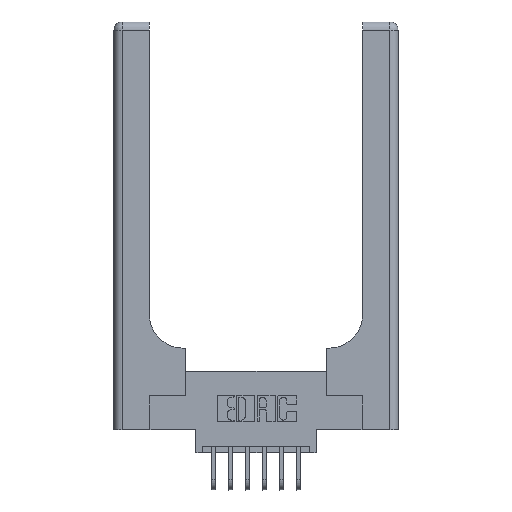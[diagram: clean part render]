
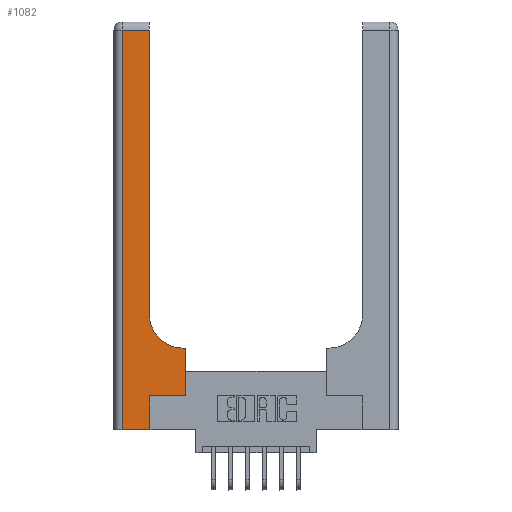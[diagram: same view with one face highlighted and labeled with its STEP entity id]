
A CAD part, top view. The second image highlights one B-rep face of the part: STEP entity #1082.
In plain terms, the highlighted planar face has unit normal (0, 0, 1).
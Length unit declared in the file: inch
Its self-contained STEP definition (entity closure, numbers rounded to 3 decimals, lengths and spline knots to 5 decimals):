
#309 = DIRECTION ( 'NONE',  ( 0., 1., 0. ) ) ;
#491 = VERTEX_POINT ( 'NONE', #1071 ) ;
#623 = CARTESIAN_POINT ( 'NONE',  ( 0.26, 0.6, 0.37 ) ) ;
#721 = VERTEX_POINT ( 'NONE', #13279 ) ;
#834 = VERTEX_POINT ( 'NONE', #8937 ) ;
#1071 = CARTESIAN_POINT ( 'NONE',  ( 0.265, 0., 0.37 ) ) ;
#1082 = ADVANCED_FACE ( 'NONE', ( #6089 ), #9531, .F. ) ;
#1418 = EDGE_CURVE ( 'NONE', #7319, #491, #8846, .T. ) ;
#1463 = CARTESIAN_POINT ( 'NONE',  ( 0.06, 0., 0.37 ) ) ;
#1487 = VERTEX_POINT ( 'NONE', #11253 ) ;
#1862 = LINE ( 'NONE', #623, #5263 ) ;
#1983 = DIRECTION ( 'NONE',  ( 0., 1., 0. ) ) ;
#2065 = ORIENTED_EDGE ( 'NONE', *, *, #6370, .T. ) ;
#2324 = CARTESIAN_POINT ( 'NONE',  ( 0., 0., 0.37 ) ) ;
#2545 = LINE ( 'NONE', #10691, #12648 ) ;
#2565 = CARTESIAN_POINT ( 'NONE',  ( 0.26, 2.94, 0.37 ) ) ;
#2700 = CARTESIAN_POINT ( 'NONE',  ( 0.51, 0.85, 0.37 ) ) ;
#2993 = VECTOR ( 'NONE', #1983, 39.37008 ) ;
#3529 = EDGE_LOOP ( 'NONE', ( #7942, #12795, #2065, #12163, #14147, #13227, #5135, #6977, #7064 ) ) ;
#3556 = EDGE_CURVE ( 'NONE', #11190, #4282, #9987, .T. ) ;
#3910 = CARTESIAN_POINT ( 'NONE',  ( 0., 2.94, 0.37 ) ) ;
#4066 = AXIS2_PLACEMENT_3D ( 'NONE', #2700, #4869, #8284 ) ;
#4282 = VERTEX_POINT ( 'NONE', #2565 ) ;
#4548 = CARTESIAN_POINT ( 'NONE',  ( 0.265, 0.25, 0.37 ) ) ;
#4570 = CARTESIAN_POINT ( 'NONE',  ( 0.26, 0.85, 0.37 ) ) ;
#4713 = EDGE_CURVE ( 'NONE', #12935, #13186, #2545, .T. ) ;
#4869 = DIRECTION ( 'NONE',  ( 0., 0., -1. ) ) ;
#5038 = DIRECTION ( 'NONE',  ( -1., 0., 0. ) ) ;
#5135 = ORIENTED_EDGE ( 'NONE', *, *, #11935, .T. ) ;
#5233 = LINE ( 'NONE', #7422, #2993 ) ;
#5263 = VECTOR ( 'NONE', #5038, 39.37008 ) ;
#5474 = DIRECTION ( 'NONE',  ( 0., 1., 0. ) ) ;
#5611 = VECTOR ( 'NONE', #14359, 39.37008 ) ;
#5801 = LINE ( 'NONE', #12477, #6898 ) ;
#5867 = CARTESIAN_POINT ( 'NONE',  ( 0., 3., 0.37 ) ) ;
#6089 = FACE_OUTER_BOUND ( 'NONE', #3529, .T. ) ;
#6301 = VECTOR ( 'NONE', #5474, 39.37008 ) ;
#6370 = EDGE_CURVE ( 'NONE', #1487, #7319, #9375, .T. ) ;
#6407 = EDGE_CURVE ( 'NONE', #721, #11190, #8878, .T. ) ;
#6898 = VECTOR ( 'NONE', #309, 39.37008 ) ;
#6977 = ORIENTED_EDGE ( 'NONE', *, *, #10795, .T. ) ;
#7064 = ORIENTED_EDGE ( 'NONE', *, *, #6407, .T. ) ;
#7268 = CARTESIAN_POINT ( 'NONE',  ( 0.06, 3., 0.37 ) ) ;
#7319 = VERTEX_POINT ( 'NONE', #1463 ) ;
#7422 = CARTESIAN_POINT ( 'NONE',  ( 0.265, 0., 0.37 ) ) ;
#7942 = ORIENTED_EDGE ( 'NONE', *, *, #3556, .T. ) ;
#8284 = DIRECTION ( 'NONE',  ( 1., 0., 0. ) ) ;
#8568 = AXIS2_PLACEMENT_3D ( 'NONE', #5867, #14009, #10554 ) ;
#8846 = LINE ( 'NONE', #2324, #5611 ) ;
#8878 = CIRCLE ( 'NONE', #4066, 0.25 ) ;
#8937 = CARTESIAN_POINT ( 'NONE',  ( 0.528, 0.6, 0.37 ) ) ;
#9375 = LINE ( 'NONE', #7268, #10310 ) ;
#9495 = DIRECTION ( 'NONE',  ( -1., 0., 0. ) ) ;
#9531 = PLANE ( 'NONE',  #8568 ) ;
#9631 = LINE ( 'NONE', #3910, #12496 ) ;
#9987 = LINE ( 'NONE', #12064, #6301 ) ;
#10310 = VECTOR ( 'NONE', #13935, 39.37008 ) ;
#10384 = EDGE_CURVE ( 'NONE', #4282, #1487, #9631, .T. ) ;
#10554 = DIRECTION ( 'NONE',  ( -1., 0., 0. ) ) ;
#10615 = DIRECTION ( 'NONE',  ( 1., 0., 0. ) ) ;
#10691 = CARTESIAN_POINT ( 'NONE',  ( 0.265, 0.25, 0.37 ) ) ;
#10795 = EDGE_CURVE ( 'NONE', #834, #721, #1862, .T. ) ;
#11190 = VERTEX_POINT ( 'NONE', #4570 ) ;
#11253 = CARTESIAN_POINT ( 'NONE',  ( 0.06, 2.94, 0.37 ) ) ;
#11935 = EDGE_CURVE ( 'NONE', #13186, #834, #5801, .T. ) ;
#12064 = CARTESIAN_POINT ( 'NONE',  ( 0.26, 3., 0.37 ) ) ;
#12102 = EDGE_CURVE ( 'NONE', #491, #12935, #5233, .T. ) ;
#12163 = ORIENTED_EDGE ( 'NONE', *, *, #1418, .T. ) ;
#12477 = CARTESIAN_POINT ( 'NONE',  ( 0.528, 0.25, 0.37 ) ) ;
#12496 = VECTOR ( 'NONE', #9495, 39.37008 ) ;
#12648 = VECTOR ( 'NONE', #10615, 39.37008 ) ;
#12795 = ORIENTED_EDGE ( 'NONE', *, *, #10384, .T. ) ;
#12935 = VERTEX_POINT ( 'NONE', #4548 ) ;
#13186 = VERTEX_POINT ( 'NONE', #13889 ) ;
#13227 = ORIENTED_EDGE ( 'NONE', *, *, #4713, .T. ) ;
#13279 = CARTESIAN_POINT ( 'NONE',  ( 0.51, 0.6, 0.37 ) ) ;
#13889 = CARTESIAN_POINT ( 'NONE',  ( 0.528, 0.25, 0.37 ) ) ;
#13935 = DIRECTION ( 'NONE',  ( 0., -1., 0. ) ) ;
#14009 = DIRECTION ( 'NONE',  ( 0., 0., -1. ) ) ;
#14147 = ORIENTED_EDGE ( 'NONE', *, *, #12102, .T. ) ;
#14359 = DIRECTION ( 'NONE',  ( 1., 0., 0. ) ) ;
